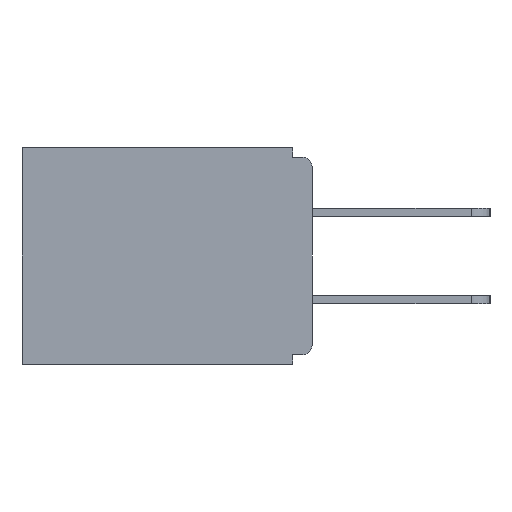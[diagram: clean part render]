
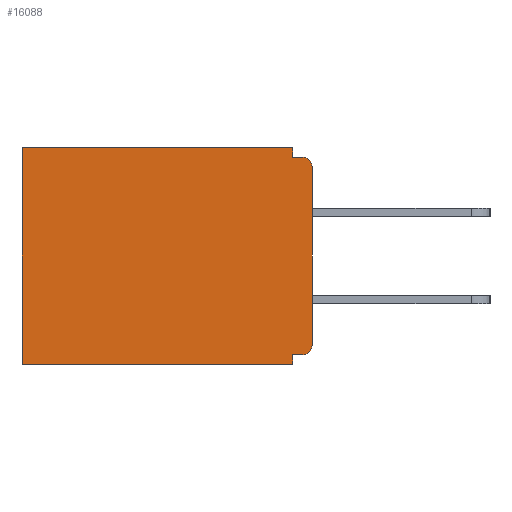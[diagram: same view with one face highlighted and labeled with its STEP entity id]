
A CAD part, left-side view. The second image highlights one B-rep face of the part: STEP entity #16088.
In plain terms, the highlighted planar face has unit normal (-1, 0, 0).
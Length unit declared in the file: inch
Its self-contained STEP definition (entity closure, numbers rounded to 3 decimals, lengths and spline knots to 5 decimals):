
#178 = ORIENTED_EDGE ( 'NONE', *, *, #5191, .F. ) ;
#802 = CARTESIAN_POINT ( 'NONE',  ( 0.298, 0., 0. ) ) ;
#1237 = ORIENTED_EDGE ( 'NONE', *, *, #21847, .T. ) ;
#2053 = EDGE_CURVE ( 'NONE', #15967, #16570, #13332, .T. ) ;
#2315 = CARTESIAN_POINT ( 'NONE',  ( 0.298, 0., -0.03 ) ) ;
#2670 = LINE ( 'NONE', #14633, #24895 ) ;
#2704 = LINE ( 'NONE', #24956, #3731 ) ;
#3435 = DIRECTION ( 'NONE',  ( -1., 0., 0. ) ) ;
#3720 = DIRECTION ( 'NONE',  ( 0., 0., -1. ) ) ;
#3731 = VECTOR ( 'NONE', #22742, 39.37008 ) ;
#4003 = CARTESIAN_POINT ( 'NONE',  ( 0.298, 0.46, 0. ) ) ;
#4470 = VECTOR ( 'NONE', #4976, 39.37008 ) ;
#4976 = DIRECTION ( 'NONE',  ( 0., 1., 0. ) ) ;
#5132 = VECTOR ( 'NONE', #10838, 39.37008 ) ;
#5191 = EDGE_CURVE ( 'NONE', #9557, #25763, #2704, .T. ) ;
#5557 = CARTESIAN_POINT ( 'NONE',  ( 0.298, 0.031, -0.328 ) ) ;
#5808 = LINE ( 'NONE', #17271, #5132 ) ;
#6310 = AXIS2_PLACEMENT_3D ( 'NONE', #12339, #3435, #3720 ) ;
#6601 = EDGE_CURVE ( 'NONE', #11787, #25817, #5808, .T. ) ;
#7146 = ORIENTED_EDGE ( 'NONE', *, *, #25785, .F. ) ;
#8160 = AXIS2_PLACEMENT_3D ( 'NONE', #18961, #21139, #8278 ) ;
#8278 = DIRECTION ( 'NONE',  ( 0., 0., -1. ) ) ;
#8339 = EDGE_CURVE ( 'NONE', #16570, #10349, #2670, .T. ) ;
#8736 = PLANE ( 'NONE',  #24184 ) ;
#9518 = DIRECTION ( 'NONE',  ( 0., 0., -1. ) ) ;
#9557 = VERTEX_POINT ( 'NONE', #12929 ) ;
#9729 = EDGE_CURVE ( 'NONE', #14897, #20435, #17084, .T. ) ;
#9815 = ORIENTED_EDGE ( 'NONE', *, *, #2053, .F. ) ;
#10007 = DIRECTION ( 'NONE',  ( 0., 0., -1. ) ) ;
#10259 = LINE ( 'NONE', #17499, #4470 ) ;
#10349 = VERTEX_POINT ( 'NONE', #18357 ) ;
#10838 = DIRECTION ( 'NONE',  ( 0., 0., -1. ) ) ;
#10902 = DIRECTION ( 'NONE',  ( 0., 0., -1. ) ) ;
#11398 = DIRECTION ( 'NONE',  ( 0., 1., 0. ) ) ;
#11787 = VERTEX_POINT ( 'NONE', #4003 ) ;
#12339 = CARTESIAN_POINT ( 'NONE',  ( 0.298, 0.015, -0.03 ) ) ;
#12929 = CARTESIAN_POINT ( 'NONE',  ( 0.298, 0.015, -0.328 ) ) ;
#13021 = ORIENTED_EDGE ( 'NONE', *, *, #22231, .T. ) ;
#13233 = CIRCLE ( 'NONE', #6310, 0.015 ) ;
#13332 = LINE ( 'NONE', #15689, #15699 ) ;
#14334 = EDGE_CURVE ( 'NONE', #9557, #20435, #26067, .T. ) ;
#14417 = LINE ( 'NONE', #27099, #20441 ) ;
#14633 = CARTESIAN_POINT ( 'NONE',  ( 0.298, 0., -0.015 ) ) ;
#14805 = CARTESIAN_POINT ( 'NONE',  ( 0.298, 0., 0. ) ) ;
#14897 = VERTEX_POINT ( 'NONE', #2315 ) ;
#15689 = CARTESIAN_POINT ( 'NONE',  ( 0.298, 0.031, -0.343 ) ) ;
#15699 = VECTOR ( 'NONE', #9518, 39.37008 ) ;
#15967 = VERTEX_POINT ( 'NONE', #20833 ) ;
#16088 = ADVANCED_FACE ( 'NONE', ( #25676 ), #8736, .F. ) ;
#16570 = VERTEX_POINT ( 'NONE', #26998 ) ;
#17084 = LINE ( 'NONE', #17291, #20450 ) ;
#17271 = CARTESIAN_POINT ( 'NONE',  ( 0.298, 0.46, 0. ) ) ;
#17291 = CARTESIAN_POINT ( 'NONE',  ( 0.298, 0., 0. ) ) ;
#17482 = ORIENTED_EDGE ( 'NONE', *, *, #14334, .T. ) ;
#17499 = CARTESIAN_POINT ( 'NONE',  ( 0.298, 0., -0.343 ) ) ;
#18357 = CARTESIAN_POINT ( 'NONE',  ( 0.298, 0.015, -0.015 ) ) ;
#18360 = ORIENTED_EDGE ( 'NONE', *, *, #8339, .F. ) ;
#18961 = CARTESIAN_POINT ( 'NONE',  ( 0.298, 0.015, -0.313 ) ) ;
#19222 = DIRECTION ( 'NONE',  ( 1., 0., 0. ) ) ;
#19716 = ORIENTED_EDGE ( 'NONE', *, *, #6601, .T. ) ;
#20435 = VERTEX_POINT ( 'NONE', #23275 ) ;
#20441 = VECTOR ( 'NONE', #10007, 39.37008 ) ;
#20450 = VECTOR ( 'NONE', #21550, 39.37008 ) ;
#20833 = CARTESIAN_POINT ( 'NONE',  ( 0.298, 0.031, 0. ) ) ;
#21139 = DIRECTION ( 'NONE',  ( -1., 0., 0. ) ) ;
#21315 = CARTESIAN_POINT ( 'NONE',  ( 0.298, 0.46, -0.343 ) ) ;
#21521 = VERTEX_POINT ( 'NONE', #26933 ) ;
#21550 = DIRECTION ( 'NONE',  ( 0., 0., -1. ) ) ;
#21576 = ORIENTED_EDGE ( 'NONE', *, *, #9729, .F. ) ;
#21599 = EDGE_CURVE ( 'NONE', #21521, #25817, #10259, .T. ) ;
#21847 = EDGE_CURVE ( 'NONE', #14897, #10349, #13233, .T. ) ;
#22231 = EDGE_CURVE ( 'NONE', #15967, #11787, #23645, .T. ) ;
#22705 = EDGE_LOOP ( 'NONE', ( #1237, #18360, #9815, #13021, #19716, #26655, #7146, #178, #17482, #21576 ) ) ;
#22742 = DIRECTION ( 'NONE',  ( 0., 1., 0. ) ) ;
#23275 = CARTESIAN_POINT ( 'NONE',  ( 0.298, 0., -0.313 ) ) ;
#23645 = LINE ( 'NONE', #802, #24294 ) ;
#24184 = AXIS2_PLACEMENT_3D ( 'NONE', #14805, #19222, #10902 ) ;
#24294 = VECTOR ( 'NONE', #11398, 39.37008 ) ;
#24895 = VECTOR ( 'NONE', #25520, 39.37008 ) ;
#24956 = CARTESIAN_POINT ( 'NONE',  ( 0.298, 0., -0.328 ) ) ;
#25520 = DIRECTION ( 'NONE',  ( 0., -1., 0. ) ) ;
#25676 = FACE_OUTER_BOUND ( 'NONE', #22705, .T. ) ;
#25763 = VERTEX_POINT ( 'NONE', #5557 ) ;
#25785 = EDGE_CURVE ( 'NONE', #25763, #21521, #14417, .T. ) ;
#25817 = VERTEX_POINT ( 'NONE', #21315 ) ;
#26067 = CIRCLE ( 'NONE', #8160, 0.015 ) ;
#26655 = ORIENTED_EDGE ( 'NONE', *, *, #21599, .F. ) ;
#26933 = CARTESIAN_POINT ( 'NONE',  ( 0.298, 0.031, -0.343 ) ) ;
#26998 = CARTESIAN_POINT ( 'NONE',  ( 0.298, 0.031, -0.015 ) ) ;
#27099 = CARTESIAN_POINT ( 'NONE',  ( 0.298, 0.031, -0.343 ) ) ;
